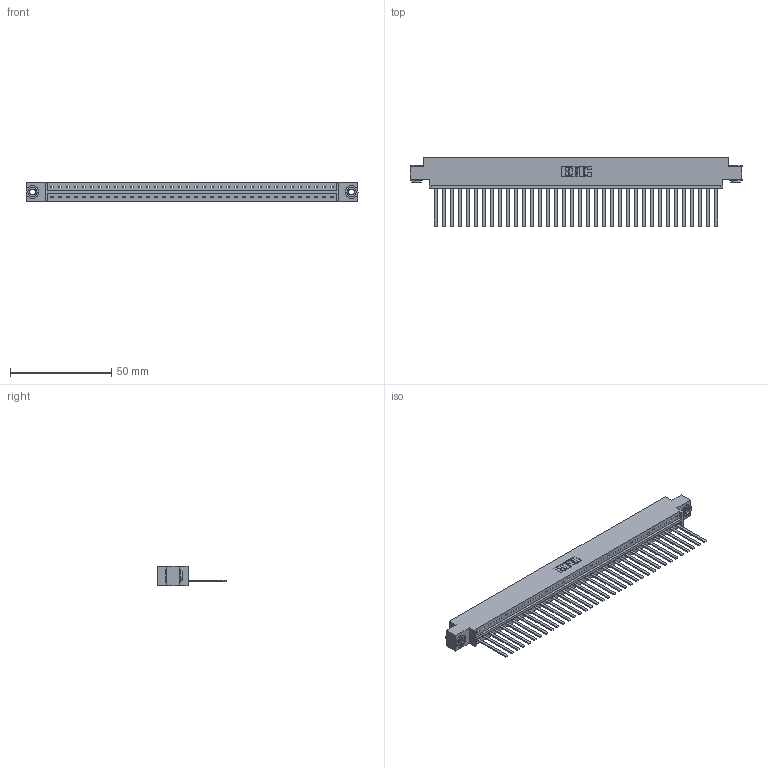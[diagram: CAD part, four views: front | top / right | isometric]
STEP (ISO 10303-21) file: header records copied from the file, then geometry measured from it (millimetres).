
FILE_DESCRIPTION (( 'STEP AP203' ), '1' );
FILE_NAME ('333-036-544-603.STEP', '2018-08-03T01:26:04', ( '' ), ( '' ), 'SwSTEP 2.0', 'SolidWorks 2016', '' );
FILE_SCHEMA (( 'CONFIG_CONTROL_DESIGN' ));
Length unit declared in the file: inch
Products named in the file (4): 345-250-002_345-250-002-102; 333-036-544-603; 333 Part_Offset - .156 Dia - TH; 345-292-001_345-293-144
Assembly tree (39 placements, depth 2):
  333-036-544-603
    333 Part_Offset - .156 Dia - TH
    345-292-001_345-293-144  x36
    345-250-002_345-250-002-102  x2
Bounding box: 164.19 x 34.3 x 9.4 mm (x, y, z)
Volume: 16678.6 mm3; surface area: 19788 mm2
Topology: 39 solids, 39 shells, 2028 faces, 6087 edges, 4006 vertices
Faces by surface type: plane 1452, cylinder 568, cone 8
Entity records: 23382 total; most frequent: CARTESIAN_POINT 4013, ORIENTED_EDGE 3978, DIRECTION 3427, EDGE_CURVE 1989, VECTOR 1841, LINE 1841, VERTEX_POINT 1322, AXIS2_PLACEMENT_3D 793
